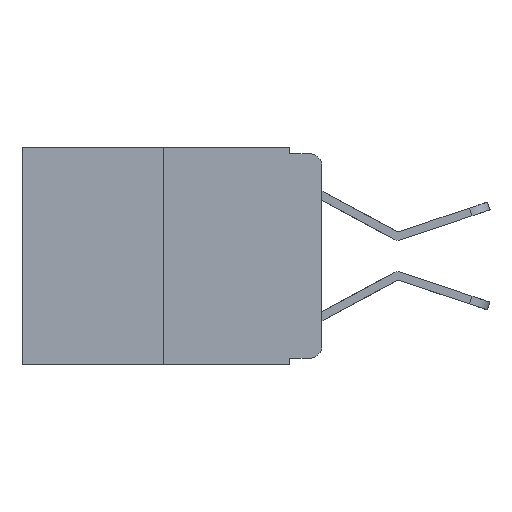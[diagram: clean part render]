
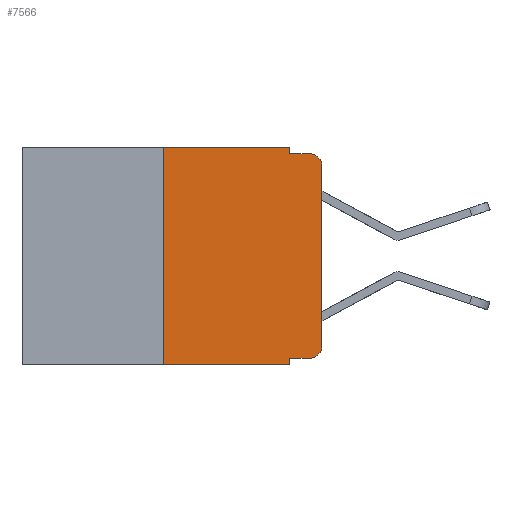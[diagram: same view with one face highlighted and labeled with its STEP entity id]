
A CAD part, left-side view. The second image highlights one B-rep face of the part: STEP entity #7566.
In plain terms, the highlighted planar face has unit normal (-1, 0, 0).
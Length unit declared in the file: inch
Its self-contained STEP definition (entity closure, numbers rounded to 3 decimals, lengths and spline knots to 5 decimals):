
#316 = CARTESIAN_POINT ( 'NONE',  ( 0., 0.02, -0.313 ) ) ;
#645 = ORIENTED_EDGE ( 'NONE', *, *, #5981, .T. ) ;
#1474 = VECTOR ( 'NONE', #16584, 39.37008 ) ;
#1480 = VERTEX_POINT ( 'NONE', #14485 ) ;
#1860 = EDGE_CURVE ( 'NONE', #21693, #1480, #6498, .T. ) ;
#2230 = DIRECTION ( 'NONE',  ( 0., 0., -1. ) ) ;
#2372 = DIRECTION ( 'NONE',  ( 0., 0., -1. ) ) ;
#2391 = AXIS2_PLACEMENT_3D ( 'NONE', #18796, #13462, #2372 ) ;
#2399 = VECTOR ( 'NONE', #18031, 39.37008 ) ;
#3573 = DIRECTION ( 'NONE',  ( 0., 0., 1. ) ) ;
#3600 = DIRECTION ( 'NONE',  ( 0., 0., -1. ) ) ;
#4124 = LINE ( 'NONE', #16432, #13351 ) ;
#4671 = VERTEX_POINT ( 'NONE', #6746 ) ;
#5081 = DIRECTION ( 'NONE',  ( -1., 0., 0. ) ) ;
#5685 = VERTEX_POINT ( 'NONE', #18688 ) ;
#5894 = ORIENTED_EDGE ( 'NONE', *, *, #23375, .T. ) ;
#5981 = EDGE_CURVE ( 'NONE', #5685, #18682, #11354, .T. ) ;
#6120 = EDGE_CURVE ( 'NONE', #21362, #8632, #4124, .T. ) ;
#6124 = ORIENTED_EDGE ( 'NONE', *, *, #1860, .F. ) ;
#6367 = CIRCLE ( 'NONE', #19003, 0.02 ) ;
#6442 = EDGE_CURVE ( 'NONE', #1480, #18682, #16163, .T. ) ;
#6460 = VECTOR ( 'NONE', #15484, 39.37008 ) ;
#6498 = LINE ( 'NONE', #13859, #1474 ) ;
#6693 = FACE_OUTER_BOUND ( 'NONE', #21560, .T. ) ;
#6746 = CARTESIAN_POINT ( 'NONE',  ( 0., 0.02, -0.333 ) ) ;
#6872 = ORIENTED_EDGE ( 'NONE', *, *, #17179, .F. ) ;
#7333 = CARTESIAN_POINT ( 'NONE',  ( 0., 0.051, -0.343 ) ) ;
#7566 = ADVANCED_FACE ( 'NONE', ( #6693 ), #22350, .F. ) ;
#8083 = VECTOR ( 'NONE', #22785, 39.37008 ) ;
#8382 = ORIENTED_EDGE ( 'NONE', *, *, #19087, .T. ) ;
#8632 = VERTEX_POINT ( 'NONE', #7333 ) ;
#9061 = EDGE_CURVE ( 'NONE', #21362, #4671, #21872, .T. ) ;
#9298 = ORIENTED_EDGE ( 'NONE', *, *, #6442, .F. ) ;
#9352 = CARTESIAN_POINT ( 'NONE',  ( 0., 0.02, -0.01 ) ) ;
#10216 = CARTESIAN_POINT ( 'NONE',  ( 0., 0.25, 0. ) ) ;
#10605 = DIRECTION ( 'NONE',  ( 0., -1., 0. ) ) ;
#10738 = ORIENTED_EDGE ( 'NONE', *, *, #9061, .T. ) ;
#11354 = CIRCLE ( 'NONE', #20981, 0.02 ) ;
#11504 = EDGE_CURVE ( 'NONE', #4671, #13791, #6367, .T. ) ;
#11589 = DIRECTION ( 'NONE',  ( 0., -1., 0. ) ) ;
#12280 = EDGE_CURVE ( 'NONE', #20172, #16154, #17707, .T. ) ;
#12354 = VECTOR ( 'NONE', #11589, 39.37008 ) ;
#12593 = CARTESIAN_POINT ( 'NONE',  ( 0., 0.473, 0. ) ) ;
#12762 = LINE ( 'NONE', #21358, #18107 ) ;
#13070 = ORIENTED_EDGE ( 'NONE', *, *, #6120, .F. ) ;
#13323 = DIRECTION ( 'NONE',  ( -1., 0., 0. ) ) ;
#13351 = VECTOR ( 'NONE', #3600, 39.37008 ) ;
#13462 = DIRECTION ( 'NONE',  ( 1., 0., 0. ) ) ;
#13654 = CARTESIAN_POINT ( 'NONE',  ( 0., 0.051, -0.01 ) ) ;
#13791 = VERTEX_POINT ( 'NONE', #19781 ) ;
#13859 = CARTESIAN_POINT ( 'NONE',  ( 0., 0.051, 0. ) ) ;
#14485 = CARTESIAN_POINT ( 'NONE',  ( 0., 0.051, -0.01 ) ) ;
#15034 = CARTESIAN_POINT ( 'NONE',  ( 0., 0.25, 0. ) ) ;
#15484 = DIRECTION ( 'NONE',  ( 0., -1., 0. ) ) ;
#16053 = CARTESIAN_POINT ( 'NONE',  ( 0., 0.02, -0.03 ) ) ;
#16154 = VERTEX_POINT ( 'NONE', #15034 ) ;
#16163 = LINE ( 'NONE', #13654, #6460 ) ;
#16432 = CARTESIAN_POINT ( 'NONE',  ( 0., 0.051, 0. ) ) ;
#16584 = DIRECTION ( 'NONE',  ( 0., 0., -1. ) ) ;
#16776 = ORIENTED_EDGE ( 'NONE', *, *, #11504, .T. ) ;
#16983 = CARTESIAN_POINT ( 'NONE',  ( 0., 0.051, 0. ) ) ;
#17179 = EDGE_CURVE ( 'NONE', #16154, #21693, #21775, .T. ) ;
#17707 = LINE ( 'NONE', #10216, #8083 ) ;
#17831 = DIRECTION ( 'NONE',  ( 0., 0., -1. ) ) ;
#18031 = DIRECTION ( 'NONE',  ( 0., -1., 0. ) ) ;
#18107 = VECTOR ( 'NONE', #10605, 39.37008 ) ;
#18115 = CARTESIAN_POINT ( 'NONE',  ( 0., 0., 0. ) ) ;
#18559 = ORIENTED_EDGE ( 'NONE', *, *, #12280, .F. ) ;
#18589 = VECTOR ( 'NONE', #3573, 39.37008 ) ;
#18682 = VERTEX_POINT ( 'NONE', #9352 ) ;
#18688 = CARTESIAN_POINT ( 'NONE',  ( 0., 0., -0.03 ) ) ;
#18760 = CARTESIAN_POINT ( 'NONE',  ( 0., 0.051, -0.333 ) ) ;
#18796 = CARTESIAN_POINT ( 'NONE',  ( 0., 0.473, 0. ) ) ;
#19003 = AXIS2_PLACEMENT_3D ( 'NONE', #316, #13323, #2230 ) ;
#19087 = EDGE_CURVE ( 'NONE', #20172, #8632, #12762, .T. ) ;
#19131 = LINE ( 'NONE', #18115, #18589 ) ;
#19781 = CARTESIAN_POINT ( 'NONE',  ( 0., 0., -0.313 ) ) ;
#20172 = VERTEX_POINT ( 'NONE', #22645 ) ;
#20981 = AXIS2_PLACEMENT_3D ( 'NONE', #16053, #5081, #17831 ) ;
#21358 = CARTESIAN_POINT ( 'NONE',  ( 0., 0.473, -0.343 ) ) ;
#21362 = VERTEX_POINT ( 'NONE', #21409 ) ;
#21409 = CARTESIAN_POINT ( 'NONE',  ( 0., 0.051, -0.333 ) ) ;
#21560 = EDGE_LOOP ( 'NONE', ( #5894, #645, #9298, #6124, #6872, #18559, #8382, #13070, #10738, #16776 ) ) ;
#21693 = VERTEX_POINT ( 'NONE', #16983 ) ;
#21775 = LINE ( 'NONE', #12593, #2399 ) ;
#21872 = LINE ( 'NONE', #18760, #12354 ) ;
#22350 = PLANE ( 'NONE',  #2391 ) ;
#22645 = CARTESIAN_POINT ( 'NONE',  ( 0., 0.25, -0.343 ) ) ;
#22785 = DIRECTION ( 'NONE',  ( 0., 0., 1. ) ) ;
#23375 = EDGE_CURVE ( 'NONE', #13791, #5685, #19131, .T. ) ;
